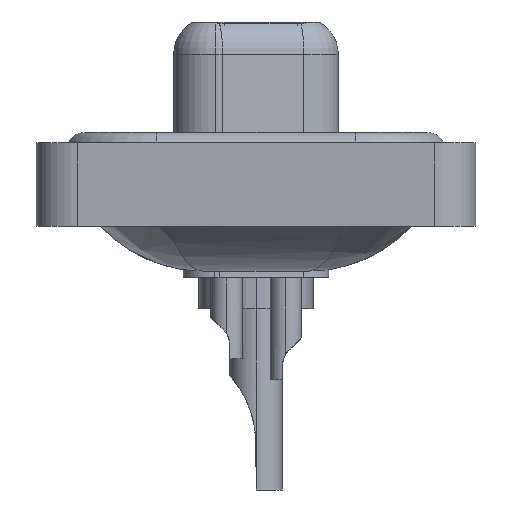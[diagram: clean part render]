
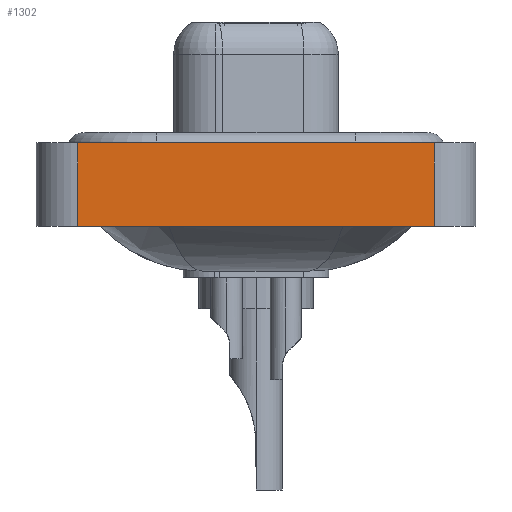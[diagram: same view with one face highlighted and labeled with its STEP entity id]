
A CAD part, left-side view. The second image highlights one B-rep face of the part: STEP entity #1302.
In plain terms, the highlighted planar face has unit normal (-1, 0, 0).
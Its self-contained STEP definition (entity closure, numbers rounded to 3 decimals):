
#361 = ORIENTED_EDGE ( 'NONE', *, *, #12250, .T. ) ;
#986 = LINE ( 'NONE', #18083, #2274 ) ;
#1158 = CARTESIAN_POINT ( 'NONE',  ( -7.25, -8.55, -3.6 ) ) ;
#1302 = ADVANCED_FACE ( 'NONE', ( #13542 ), #8818, .T. ) ;
#1450 = CARTESIAN_POINT ( 'NONE',  ( -7.25, -8.55, -3.6 ) ) ;
#1894 = VERTEX_POINT ( 'NONE', #1158 ) ;
#1913 = CARTESIAN_POINT ( 'NONE',  ( -7.25, 8.55, 0.4 ) ) ;
#1958 = ORIENTED_EDGE ( 'NONE', *, *, #14527, .T. ) ;
#2274 = VECTOR ( 'NONE', #5492, 1000. ) ;
#2580 = DIRECTION ( 'NONE',  ( -1., 0., 0. ) ) ;
#2693 = DIRECTION ( 'NONE',  ( 0., 0., 1. ) ) ;
#4231 = EDGE_CURVE ( 'NONE', #7012, #12369, #12044, .T. ) ;
#4360 = DIRECTION ( 'NONE',  ( 0., 0., 1. ) ) ;
#4718 = LINE ( 'NONE', #1450, #16872 ) ;
#5492 = DIRECTION ( 'NONE',  ( 0., 0., 1. ) ) ;
#6524 = ORIENTED_EDGE ( 'NONE', *, *, #10431, .F. ) ;
#7012 = VERTEX_POINT ( 'NONE', #1913 ) ;
#8818 = PLANE ( 'NONE',  #13134 ) ;
#8937 = CARTESIAN_POINT ( 'NONE',  ( -7.25, -8.55, -3.6 ) ) ;
#9090 = DIRECTION ( 'NONE',  ( 0., -1., 0. ) ) ;
#10386 = CARTESIAN_POINT ( 'NONE',  ( -7.25, 8.55, -3.6 ) ) ;
#10431 = EDGE_CURVE ( 'NONE', #12566, #7012, #13369, .T. ) ;
#10524 = CARTESIAN_POINT ( 'NONE',  ( -7.25, -8.55, 0.4 ) ) ;
#10604 = CARTESIAN_POINT ( 'NONE',  ( -7.25, -8.55, 0.4 ) ) ;
#10755 = DIRECTION ( 'NONE',  ( 0., -1., 0. ) ) ;
#10871 = VECTOR ( 'NONE', #4360, 1000. ) ;
#11019 = CARTESIAN_POINT ( 'NONE',  ( -7.25, 8.55, -3.6 ) ) ;
#12044 = LINE ( 'NONE', #10524, #16156 ) ;
#12250 = EDGE_CURVE ( 'NONE', #1894, #12369, #986, .T. ) ;
#12369 = VERTEX_POINT ( 'NONE', #10604 ) ;
#12566 = VERTEX_POINT ( 'NONE', #11019 ) ;
#13134 = AXIS2_PLACEMENT_3D ( 'NONE', #8937, #2580, #2693 ) ;
#13369 = LINE ( 'NONE', #10386, #10871 ) ;
#13542 = FACE_OUTER_BOUND ( 'NONE', #17718, .T. ) ;
#14527 = EDGE_CURVE ( 'NONE', #12566, #1894, #4718, .T. ) ;
#16156 = VECTOR ( 'NONE', #9090, 1000. ) ;
#16872 = VECTOR ( 'NONE', #10755, 1000. ) ;
#17718 = EDGE_LOOP ( 'NONE', ( #361, #19198, #6524, #1958 ) ) ;
#18083 = CARTESIAN_POINT ( 'NONE',  ( -7.25, -8.55, -3.6 ) ) ;
#19198 = ORIENTED_EDGE ( 'NONE', *, *, #4231, .F. ) ;
